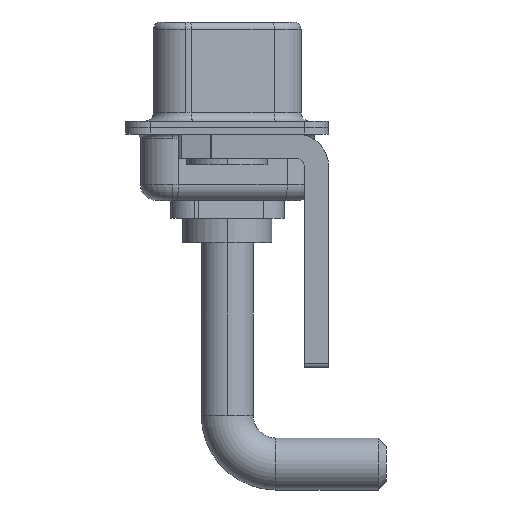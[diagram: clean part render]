
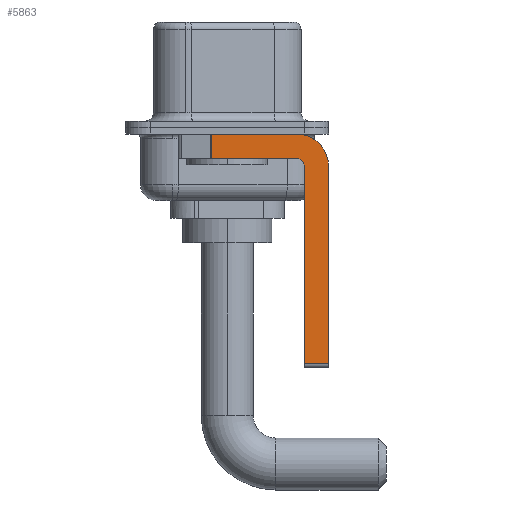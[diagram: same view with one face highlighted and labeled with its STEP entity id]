
A CAD part, left-side view. The second image highlights one B-rep face of the part: STEP entity #5863.
In plain terms, the highlighted planar face has unit normal (-1, 0, 0).
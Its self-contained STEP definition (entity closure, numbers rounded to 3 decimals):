
#524 = VERTEX_POINT ( 'NONE', #11013 ) ;
#1068 = LINE ( 'NONE', #11515, #8761 ) ;
#1207 = LINE ( 'NONE', #4746, #12280 ) ;
#1216 = DIRECTION ( 'NONE',  ( 0., 1., 0. ) ) ;
#1219 = EDGE_CURVE ( 'NONE', #12980, #3959, #1207, .T. ) ;
#1349 = CARTESIAN_POINT ( 'NONE',  ( -2.9, 0.978, -0.4 ) ) ;
#1492 = ORIENTED_EDGE ( 'NONE', *, *, #2351, .F. ) ;
#2201 = PLANE ( 'NONE',  #2774 ) ;
#2351 = EDGE_CURVE ( 'NONE', #3959, #13233, #14484, .T. ) ;
#2398 = VERTEX_POINT ( 'NONE', #4607 ) ;
#2774 = AXIS2_PLACEMENT_3D ( 'NONE', #11430, #13803, #10275 ) ;
#3302 = CARTESIAN_POINT ( 'NONE',  ( -2.9, -4.25, -2.4 ) ) ;
#3448 = DIRECTION ( 'NONE',  ( 1., 0., 0. ) ) ;
#3643 = ORIENTED_EDGE ( 'NONE', *, *, #9314, .F. ) ;
#3665 = CARTESIAN_POINT ( 'NONE',  ( -2.9, 0.978, -1.9 ) ) ;
#3959 = VERTEX_POINT ( 'NONE', #12002 ) ;
#4607 = CARTESIAN_POINT ( 'NONE',  ( -2.9, -4.75, -2.4 ) ) ;
#4660 = ORIENTED_EDGE ( 'NONE', *, *, #6592, .F. ) ;
#4677 = CARTESIAN_POINT ( 'NONE',  ( -2.9, -4.75, -14.55 ) ) ;
#4746 = CARTESIAN_POINT ( 'NONE',  ( -2.9, 3., -0.4 ) ) ;
#5299 = EDGE_CURVE ( 'NONE', #13233, #14596, #7392, .T. ) ;
#5366 = EDGE_CURVE ( 'NONE', #2398, #524, #11843, .T. ) ;
#5598 = FACE_OUTER_BOUND ( 'NONE', #10973, .T. ) ;
#5715 = ORIENTED_EDGE ( 'NONE', *, *, #5366, .F. ) ;
#5784 = ORIENTED_EDGE ( 'NONE', *, *, #1219, .F. ) ;
#5863 = ADVANCED_FACE ( 'NONE', ( #5598 ), #2201, .F. ) ;
#6592 = EDGE_CURVE ( 'NONE', #9335, #2398, #13428, .T. ) ;
#6754 = DIRECTION ( 'NONE',  ( -1., 0., 0. ) ) ;
#6856 = CARTESIAN_POINT ( 'NONE',  ( -2.9, -6.25, -2.4 ) ) ;
#6975 = CARTESIAN_POINT ( 'NONE',  ( -2.9, -4.25, -2.4 ) ) ;
#7044 = ORIENTED_EDGE ( 'NONE', *, *, #5299, .F. ) ;
#7392 = LINE ( 'NONE', #8987, #10372 ) ;
#7619 = CARTESIAN_POINT ( 'NONE',  ( -2.9, 0.978, -1.9 ) ) ;
#8147 = AXIS2_PLACEMENT_3D ( 'NONE', #3302, #6754, #9210 ) ;
#8360 = DIRECTION ( 'NONE',  ( 0., 0., -1. ) ) ;
#8444 = DIRECTION ( 'NONE',  ( 0., -1., 0. ) ) ;
#8761 = VECTOR ( 'NONE', #1216, 1000. ) ;
#8878 = DIRECTION ( 'NONE',  ( 0., 0., 1. ) ) ;
#8987 = CARTESIAN_POINT ( 'NONE',  ( -2.9, -6.25, -2.4 ) ) ;
#9210 = DIRECTION ( 'NONE',  ( 0., 0., 1. ) ) ;
#9314 = EDGE_CURVE ( 'NONE', #524, #13568, #1068, .T. ) ;
#9335 = VERTEX_POINT ( 'NONE', #4677 ) ;
#9833 = AXIS2_PLACEMENT_3D ( 'NONE', #6975, #3448, #8360 ) ;
#9935 = ORIENTED_EDGE ( 'NONE', *, *, #10907, .T. ) ;
#9961 = CARTESIAN_POINT ( 'NONE',  ( -2.9, -4.75, -14.8 ) ) ;
#10275 = DIRECTION ( 'NONE',  ( 0., 0., -1. ) ) ;
#10372 = VECTOR ( 'NONE', #11371, 1000. ) ;
#10588 = DIRECTION ( 'NONE',  ( 0., 0., -1. ) ) ;
#10748 = LINE ( 'NONE', #3665, #14904 ) ;
#10907 = EDGE_CURVE ( 'NONE', #9335, #14596, #11992, .T. ) ;
#10973 = EDGE_LOOP ( 'NONE', ( #5784, #12878, #3643, #5715, #4660, #9935, #7044, #1492 ) ) ;
#11013 = CARTESIAN_POINT ( 'NONE',  ( -2.9, -4.25, -1.9 ) ) ;
#11371 = DIRECTION ( 'NONE',  ( 0., 0., -1. ) ) ;
#11430 = CARTESIAN_POINT ( 'NONE',  ( -2.9, -4.25, -2.4 ) ) ;
#11515 = CARTESIAN_POINT ( 'NONE',  ( -2.9, -4.25, -1.9 ) ) ;
#11843 = CIRCLE ( 'NONE', #8147, 0.5 ) ;
#11992 = LINE ( 'NONE', #13144, #13933 ) ;
#12002 = CARTESIAN_POINT ( 'NONE',  ( -2.9, -4.25, -0.4 ) ) ;
#12280 = VECTOR ( 'NONE', #13962, 1000. ) ;
#12412 = CARTESIAN_POINT ( 'NONE',  ( -2.9, -6.25, -14.55 ) ) ;
#12513 = EDGE_CURVE ( 'NONE', #12980, #13568, #10748, .T. ) ;
#12878 = ORIENTED_EDGE ( 'NONE', *, *, #12513, .T. ) ;
#12980 = VERTEX_POINT ( 'NONE', #1349 ) ;
#13144 = CARTESIAN_POINT ( 'NONE',  ( -2.9, -4.25, -14.55 ) ) ;
#13233 = VERTEX_POINT ( 'NONE', #6856 ) ;
#13428 = LINE ( 'NONE', #9961, #13836 ) ;
#13568 = VERTEX_POINT ( 'NONE', #7619 ) ;
#13803 = DIRECTION ( 'NONE',  ( 1., 0., 0. ) ) ;
#13836 = VECTOR ( 'NONE', #8878, 1000. ) ;
#13933 = VECTOR ( 'NONE', #8444, 1000. ) ;
#13962 = DIRECTION ( 'NONE',  ( 0., -1., 0. ) ) ;
#14484 = CIRCLE ( 'NONE', #9833, 2. ) ;
#14596 = VERTEX_POINT ( 'NONE', #12412 ) ;
#14904 = VECTOR ( 'NONE', #10588, 1000. ) ;
